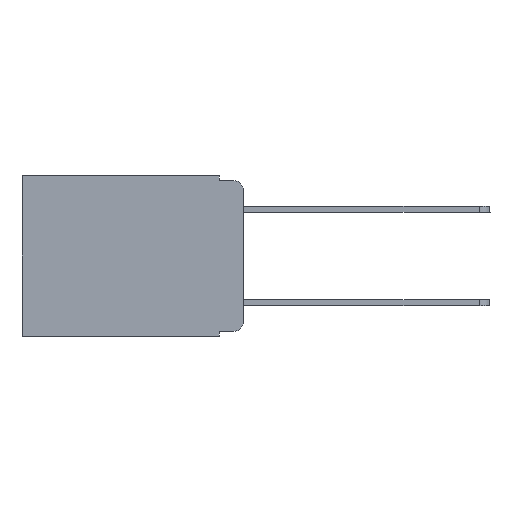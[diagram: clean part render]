
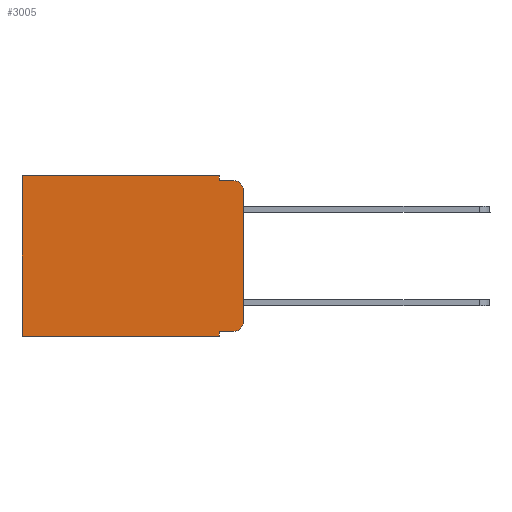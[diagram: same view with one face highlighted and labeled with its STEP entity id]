
A CAD part, left-side view. The second image highlights one B-rep face of the part: STEP entity #3005.
In plain terms, the highlighted planar face has unit normal (-1, 0, 0).
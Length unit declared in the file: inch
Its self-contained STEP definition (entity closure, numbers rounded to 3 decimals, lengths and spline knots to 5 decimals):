
#47 = LINE ( 'NONE', #7316, #166 ) ;
#140 = VECTOR ( 'NONE', #1289, 39.37008 ) ;
#166 = VECTOR ( 'NONE', #13170, 39.37008 ) ;
#361 = CIRCLE ( 'NONE', #6092, 0.02 ) ;
#372 = ORIENTED_EDGE ( 'NONE', *, *, #4069, .F. ) ;
#522 = LINE ( 'NONE', #3189, #13340 ) ;
#852 = ORIENTED_EDGE ( 'NONE', *, *, #3468, .T. ) ;
#1109 = VERTEX_POINT ( 'NONE', #5974 ) ;
#1289 = DIRECTION ( 'NONE',  ( 0., 0., -1. ) ) ;
#1911 = CARTESIAN_POINT ( 'NONE',  ( 0.298, 0.473, -0.343 ) ) ;
#3005 = ADVANCED_FACE ( 'NONE', ( #3486 ), #3392, .F. ) ;
#3165 = VERTEX_POINT ( 'NONE', #5641 ) ;
#3189 = CARTESIAN_POINT ( 'NONE',  ( 0.298, 0.051, -0.333 ) ) ;
#3236 = CARTESIAN_POINT ( 'NONE',  ( 0.298, 0.051, -0.01 ) ) ;
#3255 = CIRCLE ( 'NONE', #17117, 0.02 ) ;
#3368 = DIRECTION ( 'NONE',  ( 0., -1., 0. ) ) ;
#3392 = PLANE ( 'NONE',  #12868 ) ;
#3468 = EDGE_CURVE ( 'NONE', #10915, #8588, #522, .T. ) ;
#3486 = FACE_OUTER_BOUND ( 'NONE', #5079, .T. ) ;
#3584 = ORIENTED_EDGE ( 'NONE', *, *, #15355, .F. ) ;
#3863 = CARTESIAN_POINT ( 'NONE',  ( 0.298, 0., -0.03 ) ) ;
#4069 = EDGE_CURVE ( 'NONE', #16915, #4304, #5596, .T. ) ;
#4132 = DIRECTION ( 'NONE',  ( 0., 0., -1. ) ) ;
#4303 = DIRECTION ( 'NONE',  ( 0., 0., -1. ) ) ;
#4304 = VERTEX_POINT ( 'NONE', #3236 ) ;
#4378 = CARTESIAN_POINT ( 'NONE',  ( 0.298, 0.051, 0. ) ) ;
#4741 = VECTOR ( 'NONE', #4303, 39.37008 ) ;
#4959 = EDGE_CURVE ( 'NONE', #18537, #12508, #5621, .T. ) ;
#5079 = EDGE_LOOP ( 'NONE', ( #6140, #10300, #7281, #372, #6636, #9661, #3584, #16212, #852, #9620 ) ) ;
#5553 = CARTESIAN_POINT ( 'NONE',  ( 0.298, 0.02, -0.03 ) ) ;
#5596 = LINE ( 'NONE', #4378, #14414 ) ;
#5621 = LINE ( 'NONE', #14318, #4741 ) ;
#5641 = CARTESIAN_POINT ( 'NONE',  ( 0.298, 0.473, 0. ) ) ;
#5729 = LINE ( 'NONE', #15544, #7517 ) ;
#5974 = CARTESIAN_POINT ( 'NONE',  ( 0.298, 0.051, -0.343 ) ) ;
#6092 = AXIS2_PLACEMENT_3D ( 'NONE', #5553, #17064, #4132 ) ;
#6140 = ORIENTED_EDGE ( 'NONE', *, *, #4959, .F. ) ;
#6315 = DIRECTION ( 'NONE',  ( 0., 0., -1. ) ) ;
#6397 = EDGE_CURVE ( 'NONE', #4304, #10136, #5729, .T. ) ;
#6475 = EDGE_CURVE ( 'NONE', #10915, #1109, #8030, .T. ) ;
#6636 = ORIENTED_EDGE ( 'NONE', *, *, #13469, .T. ) ;
#6762 = CARTESIAN_POINT ( 'NONE',  ( 0.298, 0.02, -0.313 ) ) ;
#6768 = CARTESIAN_POINT ( 'NONE',  ( 0.298, 0.473, 0. ) ) ;
#7281 = ORIENTED_EDGE ( 'NONE', *, *, #6397, .F. ) ;
#7316 = CARTESIAN_POINT ( 'NONE',  ( 0.298, 0., 0. ) ) ;
#7517 = VECTOR ( 'NONE', #8365, 39.37008 ) ;
#8030 = LINE ( 'NONE', #9269, #15979 ) ;
#8278 = VERTEX_POINT ( 'NONE', #1911 ) ;
#8365 = DIRECTION ( 'NONE',  ( 0., -1., 0. ) ) ;
#8588 = VERTEX_POINT ( 'NONE', #13212 ) ;
#8841 = DIRECTION ( 'NONE',  ( 0., 0., -1. ) ) ;
#8877 = EDGE_CURVE ( 'NONE', #18537, #10136, #361, .T. ) ;
#9230 = DIRECTION ( 'NONE',  ( 1., 0., 0. ) ) ;
#9269 = CARTESIAN_POINT ( 'NONE',  ( 0.298, 0.051, 0. ) ) ;
#9620 = ORIENTED_EDGE ( 'NONE', *, *, #17402, .T. ) ;
#9661 = ORIENTED_EDGE ( 'NONE', *, *, #12910, .T. ) ;
#10136 = VERTEX_POINT ( 'NONE', #17931 ) ;
#10300 = ORIENTED_EDGE ( 'NONE', *, *, #8877, .T. ) ;
#10578 = CARTESIAN_POINT ( 'NONE',  ( 0.298, 0.051, -0.333 ) ) ;
#10750 = VECTOR ( 'NONE', #16909, 39.37008 ) ;
#10915 = VERTEX_POINT ( 'NONE', #10578 ) ;
#12508 = VERTEX_POINT ( 'NONE', #17976 ) ;
#12527 = DIRECTION ( 'NONE',  ( -1., 0., 0. ) ) ;
#12868 = AXIS2_PLACEMENT_3D ( 'NONE', #16590, #9230, #6315 ) ;
#12910 = EDGE_CURVE ( 'NONE', #3165, #8278, #15558, .T. ) ;
#13170 = DIRECTION ( 'NONE',  ( 0., 1., 0. ) ) ;
#13212 = CARTESIAN_POINT ( 'NONE',  ( 0.298, 0.02, -0.333 ) ) ;
#13340 = VECTOR ( 'NONE', #3368, 39.37008 ) ;
#13469 = EDGE_CURVE ( 'NONE', #16915, #3165, #47, .T. ) ;
#13794 = CARTESIAN_POINT ( 'NONE',  ( 0.298, 0., -0.343 ) ) ;
#14318 = CARTESIAN_POINT ( 'NONE',  ( 0.298, 0., 0. ) ) ;
#14414 = VECTOR ( 'NONE', #14470, 39.37008 ) ;
#14470 = DIRECTION ( 'NONE',  ( 0., 0., -1. ) ) ;
#15355 = EDGE_CURVE ( 'NONE', #1109, #8278, #15589, .T. ) ;
#15544 = CARTESIAN_POINT ( 'NONE',  ( 0.298, 0.051, -0.01 ) ) ;
#15558 = LINE ( 'NONE', #6768, #140 ) ;
#15589 = LINE ( 'NONE', #13794, #10750 ) ;
#15979 = VECTOR ( 'NONE', #8841, 39.37008 ) ;
#16212 = ORIENTED_EDGE ( 'NONE', *, *, #6475, .F. ) ;
#16590 = CARTESIAN_POINT ( 'NONE',  ( 0.298, 0., 0. ) ) ;
#16870 = DIRECTION ( 'NONE',  ( 0., 0., -1. ) ) ;
#16909 = DIRECTION ( 'NONE',  ( 0., 1., 0. ) ) ;
#16915 = VERTEX_POINT ( 'NONE', #16998 ) ;
#16998 = CARTESIAN_POINT ( 'NONE',  ( 0.298, 0.051, 0. ) ) ;
#17064 = DIRECTION ( 'NONE',  ( -1., 0., 0. ) ) ;
#17117 = AXIS2_PLACEMENT_3D ( 'NONE', #6762, #12527, #16870 ) ;
#17402 = EDGE_CURVE ( 'NONE', #8588, #12508, #3255, .T. ) ;
#17931 = CARTESIAN_POINT ( 'NONE',  ( 0.298, 0.02, -0.01 ) ) ;
#17976 = CARTESIAN_POINT ( 'NONE',  ( 0.298, 0., -0.313 ) ) ;
#18537 = VERTEX_POINT ( 'NONE', #3863 ) ;
